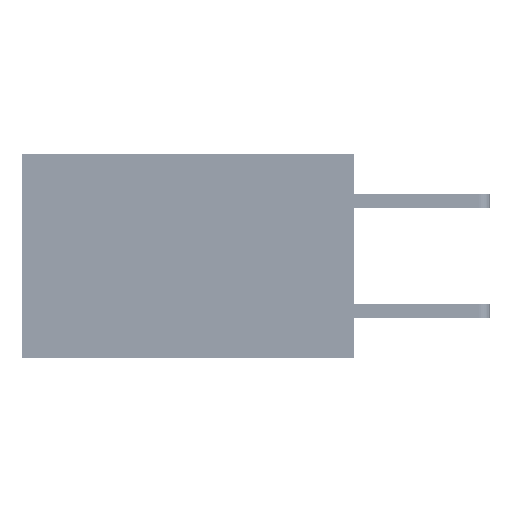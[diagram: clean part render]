
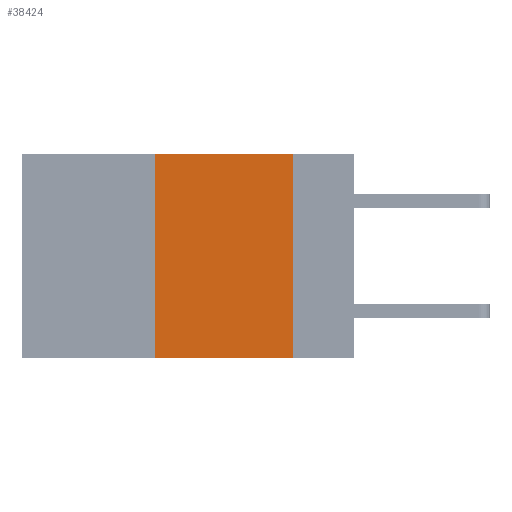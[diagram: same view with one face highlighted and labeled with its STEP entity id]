
A CAD part, left-side view. The second image highlights one B-rep face of the part: STEP entity #38424.
In plain terms, the highlighted planar face has unit normal (-1, 0, 0).
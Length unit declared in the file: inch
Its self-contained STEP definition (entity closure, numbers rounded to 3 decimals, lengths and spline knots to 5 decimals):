
#2212 = LINE ( 'NONE', #13923, #25576 ) ;
#6604 = CARTESIAN_POINT ( 'NONE',  ( 0., 0.6, 0. ) ) ;
#11012 = CARTESIAN_POINT ( 'NONE',  ( 0., 0.36, 0. ) ) ;
#11414 = CARTESIAN_POINT ( 'NONE',  ( 0., 0.36, -0.37 ) ) ;
#12436 = CARTESIAN_POINT ( 'NONE',  ( 0., 0.6, -0.37 ) ) ;
#13923 = CARTESIAN_POINT ( 'NONE',  ( 0., 0.11, 0. ) ) ;
#14017 = CARTESIAN_POINT ( 'NONE',  ( 0., 0.36, 0. ) ) ;
#14836 = LINE ( 'NONE', #11012, #30310 ) ;
#16316 = EDGE_CURVE ( 'NONE', #39765, #19924, #47382, .T. ) ;
#16508 = DIRECTION ( 'NONE',  ( 0., -1., 0. ) ) ;
#16748 = ORIENTED_EDGE ( 'NONE', *, *, #32388, .F. ) ;
#17398 = VECTOR ( 'NONE', #17872, 39.37008 ) ;
#17563 = FACE_OUTER_BOUND ( 'NONE', #23503, .T. ) ;
#17872 = DIRECTION ( 'NONE',  ( 0., -1., 0. ) ) ;
#18075 = DIRECTION ( 'NONE',  ( 0., 0., -1. ) ) ;
#19924 = VERTEX_POINT ( 'NONE', #45128 ) ;
#21470 = DIRECTION ( 'NONE',  ( 0., 0., 1. ) ) ;
#21890 = DIRECTION ( 'NONE',  ( 1., 0., 0. ) ) ;
#23503 = EDGE_LOOP ( 'NONE', ( #45394, #40093, #16748, #44794 ) ) ;
#25576 = VECTOR ( 'NONE', #29466, 39.37008 ) ;
#29333 = LINE ( 'NONE', #44912, #17398 ) ;
#29466 = DIRECTION ( 'NONE',  ( 0., 0., -1. ) ) ;
#30310 = VECTOR ( 'NONE', #21470, 39.37008 ) ;
#30650 = VECTOR ( 'NONE', #16508, 39.37008 ) ;
#32388 = EDGE_CURVE ( 'NONE', #39765, #32751, #14836, .T. ) ;
#32751 = VERTEX_POINT ( 'NONE', #14017 ) ;
#35322 = EDGE_CURVE ( 'NONE', #32751, #46540, #29333, .T. ) ;
#36050 = CARTESIAN_POINT ( 'NONE',  ( 0., 0.11, 0. ) ) ;
#38424 = ADVANCED_FACE ( 'NONE', ( #17563 ), #41546, .F. ) ;
#39765 = VERTEX_POINT ( 'NONE', #11414 ) ;
#40093 = ORIENTED_EDGE ( 'NONE', *, *, #35322, .F. ) ;
#41546 = PLANE ( 'NONE',  #41952 ) ;
#41952 = AXIS2_PLACEMENT_3D ( 'NONE', #6604, #21890, #18075 ) ;
#44794 = ORIENTED_EDGE ( 'NONE', *, *, #16316, .T. ) ;
#44912 = CARTESIAN_POINT ( 'NONE',  ( 0., 0.6, 0. ) ) ;
#45128 = CARTESIAN_POINT ( 'NONE',  ( 0., 0.11, -0.37 ) ) ;
#45394 = ORIENTED_EDGE ( 'NONE', *, *, #47623, .F. ) ;
#46540 = VERTEX_POINT ( 'NONE', #36050 ) ;
#47382 = LINE ( 'NONE', #12436, #30650 ) ;
#47623 = EDGE_CURVE ( 'NONE', #46540, #19924, #2212, .T. ) ;
